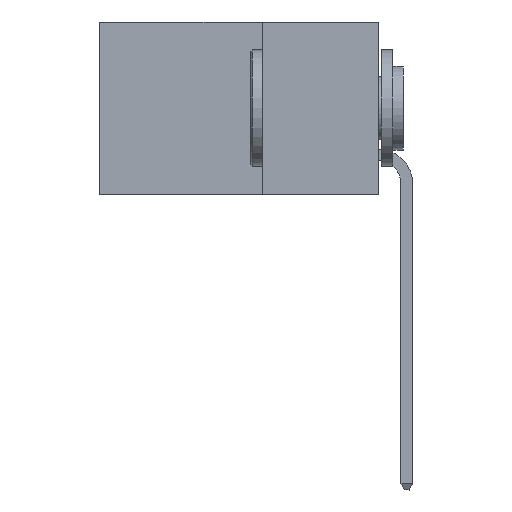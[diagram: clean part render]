
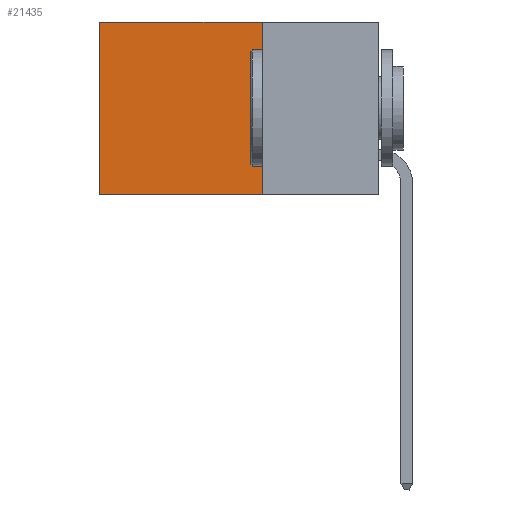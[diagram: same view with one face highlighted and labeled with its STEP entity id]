
A CAD part, left-side view. The second image highlights one B-rep face of the part: STEP entity #21435.
In plain terms, the highlighted planar face has unit normal (-1, 0, 0).
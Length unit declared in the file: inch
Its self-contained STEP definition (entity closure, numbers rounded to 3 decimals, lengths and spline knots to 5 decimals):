
#487 = PLANE ( 'NONE',  #9097 ) ;
#556 = EDGE_LOOP ( 'NONE', ( #12395, #12943, #4004, #11086 ) ) ;
#1030 = DIRECTION ( 'NONE',  ( 0., 0., -1. ) ) ;
#2533 = LINE ( 'NONE', #8678, #31634 ) ;
#2681 = CARTESIAN_POINT ( 'NONE',  ( 0.298, 0.25, -0.37 ) ) ;
#2885 = VECTOR ( 'NONE', #20427, 39.37008 ) ;
#4004 = ORIENTED_EDGE ( 'NONE', *, *, #26676, .F. ) ;
#4071 = VECTOR ( 'NONE', #16550, 39.37008 ) ;
#5029 = CARTESIAN_POINT ( 'NONE',  ( 0.298, 0.6, 0. ) ) ;
#6845 = FACE_OUTER_BOUND ( 'NONE', #556, .T. ) ;
#8678 = CARTESIAN_POINT ( 'NONE',  ( 0.298, 0.6, 0. ) ) ;
#9097 = AXIS2_PLACEMENT_3D ( 'NONE', #10434, #20418, #23182 ) ;
#9338 = VECTOR ( 'NONE', #10759, 39.37008 ) ;
#9390 = VERTEX_POINT ( 'NONE', #9567 ) ;
#9567 = CARTESIAN_POINT ( 'NONE',  ( 0.298, 0.25, 0. ) ) ;
#10434 = CARTESIAN_POINT ( 'NONE',  ( 0.298, 0.25, 0. ) ) ;
#10759 = DIRECTION ( 'NONE',  ( 0., 0., -1. ) ) ;
#11034 = VERTEX_POINT ( 'NONE', #5029 ) ;
#11086 = ORIENTED_EDGE ( 'NONE', *, *, #31390, .T. ) ;
#12395 = ORIENTED_EDGE ( 'NONE', *, *, #28776, .T. ) ;
#12943 = ORIENTED_EDGE ( 'NONE', *, *, #22288, .F. ) ;
#13191 = CARTESIAN_POINT ( 'NONE',  ( 0.298, 0.25, 0. ) ) ;
#14688 = VERTEX_POINT ( 'NONE', #28057 ) ;
#16550 = DIRECTION ( 'NONE',  ( 0., 1., 0. ) ) ;
#20418 = DIRECTION ( 'NONE',  ( 1., 0., 0. ) ) ;
#20427 = DIRECTION ( 'NONE',  ( 0., 1., 0. ) ) ;
#21435 = ADVANCED_FACE ( 'NONE', ( #6845 ), #487, .F. ) ;
#22288 = EDGE_CURVE ( 'NONE', #25547, #14688, #26516, .T. ) ;
#23182 = DIRECTION ( 'NONE',  ( 0., 0., -1. ) ) ;
#25547 = VERTEX_POINT ( 'NONE', #30813 ) ;
#26158 = LINE ( 'NONE', #31620, #4071 ) ;
#26516 = LINE ( 'NONE', #2681, #2885 ) ;
#26676 = EDGE_CURVE ( 'NONE', #9390, #25547, #31006, .T. ) ;
#28057 = CARTESIAN_POINT ( 'NONE',  ( 0.298, 0.6, -0.37 ) ) ;
#28776 = EDGE_CURVE ( 'NONE', #11034, #14688, #2533, .T. ) ;
#30813 = CARTESIAN_POINT ( 'NONE',  ( 0.298, 0.25, -0.37 ) ) ;
#31006 = LINE ( 'NONE', #13191, #9338 ) ;
#31390 = EDGE_CURVE ( 'NONE', #9390, #11034, #26158, .T. ) ;
#31620 = CARTESIAN_POINT ( 'NONE',  ( 0.298, 0.25, 0. ) ) ;
#31634 = VECTOR ( 'NONE', #1030, 39.37008 ) ;
